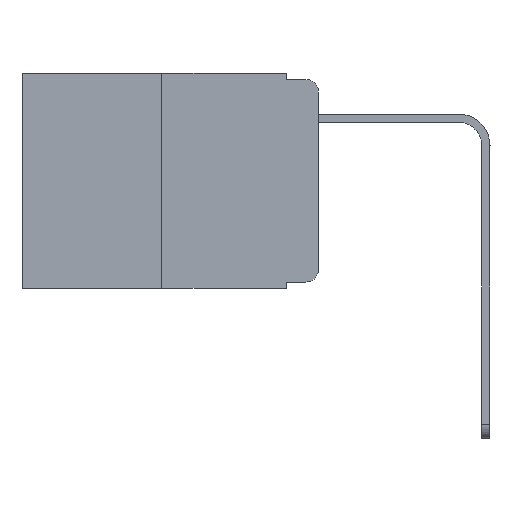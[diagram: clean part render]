
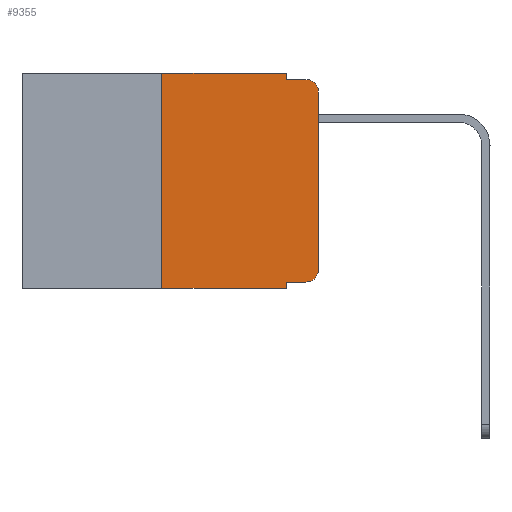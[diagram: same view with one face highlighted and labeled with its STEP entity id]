
A CAD part, left-side view. The second image highlights one B-rep face of the part: STEP entity #9355.
In plain terms, the highlighted planar face has unit normal (-1, 0, 0).
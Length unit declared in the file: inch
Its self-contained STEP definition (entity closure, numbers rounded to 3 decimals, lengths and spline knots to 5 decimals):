
#103 = VECTOR ( 'NONE', #19092, 39.37008 ) ;
#157 = EDGE_CURVE ( 'NONE', #6366, #18895, #11371, .T. ) ;
#1307 = VERTEX_POINT ( 'NONE', #1701 ) ;
#1343 = CARTESIAN_POINT ( 'NONE',  ( 0., 0.473, 0. ) ) ;
#1406 = DIRECTION ( 'NONE',  ( 0., -1., 0. ) ) ;
#1701 = CARTESIAN_POINT ( 'NONE',  ( 0., 0.25, 0. ) ) ;
#1942 = DIRECTION ( 'NONE',  ( -1., 0., 0. ) ) ;
#1989 = DIRECTION ( 'NONE',  ( -1., 0., 0. ) ) ;
#2503 = ORIENTED_EDGE ( 'NONE', *, *, #11614, .F. ) ;
#2694 = ORIENTED_EDGE ( 'NONE', *, *, #22215, .T. ) ;
#2781 = ORIENTED_EDGE ( 'NONE', *, *, #11770, .T. ) ;
#2900 = ORIENTED_EDGE ( 'NONE', *, *, #15340, .T. ) ;
#3020 = AXIS2_PLACEMENT_3D ( 'NONE', #21600, #1989, #19789 ) ;
#3275 = CARTESIAN_POINT ( 'NONE',  ( 0., 0.02, -0.333 ) ) ;
#3338 = DIRECTION ( 'NONE',  ( 0., 0., -1. ) ) ;
#3390 = LINE ( 'NONE', #14131, #22844 ) ;
#3753 = DIRECTION ( 'NONE',  ( 1., 0., 0. ) ) ;
#3938 = ORIENTED_EDGE ( 'NONE', *, *, #6670, .F. ) ;
#4120 = VECTOR ( 'NONE', #8656, 39.37008 ) ;
#4743 = AXIS2_PLACEMENT_3D ( 'NONE', #11235, #3753, #11484 ) ;
#4782 = VECTOR ( 'NONE', #10797, 39.37008 ) ;
#5432 = VECTOR ( 'NONE', #19909, 39.37008 ) ;
#5450 = ORIENTED_EDGE ( 'NONE', *, *, #157, .T. ) ;
#5679 = VERTEX_POINT ( 'NONE', #12437 ) ;
#6134 = VERTEX_POINT ( 'NONE', #3275 ) ;
#6366 = VERTEX_POINT ( 'NONE', #16719 ) ;
#6670 = EDGE_CURVE ( 'NONE', #13632, #20905, #15240, .T. ) ;
#7025 = ORIENTED_EDGE ( 'NONE', *, *, #9251, .F. ) ;
#7073 = ORIENTED_EDGE ( 'NONE', *, *, #15462, .F. ) ;
#7730 = CARTESIAN_POINT ( 'NONE',  ( 0., 0.25, -0.343 ) ) ;
#8656 = DIRECTION ( 'NONE',  ( 0., 0., -1. ) ) ;
#8911 = LINE ( 'NONE', #25001, #10462 ) ;
#9138 = EDGE_CURVE ( 'NONE', #13632, #6134, #19129, .T. ) ;
#9189 = ORIENTED_EDGE ( 'NONE', *, *, #9138, .T. ) ;
#9251 = EDGE_CURVE ( 'NONE', #23911, #1307, #3390, .T. ) ;
#9355 = ADVANCED_FACE ( 'NONE', ( #24097 ), #10888, .F. ) ;
#9690 = CARTESIAN_POINT ( 'NONE',  ( 0., 0.02, -0.03 ) ) ;
#10042 = CARTESIAN_POINT ( 'NONE',  ( 0., 0., 0. ) ) ;
#10237 = DIRECTION ( 'NONE',  ( 0., -1., 0. ) ) ;
#10462 = VECTOR ( 'NONE', #3338, 39.37008 ) ;
#10703 = CIRCLE ( 'NONE', #20778, 0.02 ) ;
#10740 = EDGE_CURVE ( 'NONE', #5679, #23069, #8911, .T. ) ;
#10797 = DIRECTION ( 'NONE',  ( 0., -1., 0. ) ) ;
#10888 = PLANE ( 'NONE',  #4743 ) ;
#11195 = CARTESIAN_POINT ( 'NONE',  ( 0., 0.051, 0. ) ) ;
#11235 = CARTESIAN_POINT ( 'NONE',  ( 0., 0.473, 0. ) ) ;
#11371 = LINE ( 'NONE', #10042, #5432 ) ;
#11484 = DIRECTION ( 'NONE',  ( 0., 0., -1. ) ) ;
#11614 = EDGE_CURVE ( 'NONE', #1307, #5679, #19893, .T. ) ;
#11694 = DIRECTION ( 'NONE',  ( 0., 0., -1. ) ) ;
#11770 = EDGE_CURVE ( 'NONE', #18895, #24451, #10703, .T. ) ;
#12437 = CARTESIAN_POINT ( 'NONE',  ( 0., 0.051, 0. ) ) ;
#12655 = VECTOR ( 'NONE', #1406, 39.37008 ) ;
#12814 = CARTESIAN_POINT ( 'NONE',  ( 0., 0.051, -0.333 ) ) ;
#13632 = VERTEX_POINT ( 'NONE', #12814 ) ;
#14131 = CARTESIAN_POINT ( 'NONE',  ( 0., 0.25, 0. ) ) ;
#15240 = LINE ( 'NONE', #11195, #4120 ) ;
#15340 = EDGE_CURVE ( 'NONE', #6134, #6366, #23103, .T. ) ;
#15462 = EDGE_CURVE ( 'NONE', #23069, #24451, #20326, .T. ) ;
#16719 = CARTESIAN_POINT ( 'NONE',  ( 0., 0., -0.313 ) ) ;
#17278 = DIRECTION ( 'NONE',  ( 0., 0., 1. ) ) ;
#17351 = CARTESIAN_POINT ( 'NONE',  ( 0., 0.051, -0.01 ) ) ;
#18026 = CARTESIAN_POINT ( 'NONE',  ( 0., 0.051, -0.343 ) ) ;
#18305 = ORIENTED_EDGE ( 'NONE', *, *, #10740, .F. ) ;
#18895 = VERTEX_POINT ( 'NONE', #23043 ) ;
#19092 = DIRECTION ( 'NONE',  ( 0., -1., 0. ) ) ;
#19129 = LINE ( 'NONE', #20832, #103 ) ;
#19789 = DIRECTION ( 'NONE',  ( 0., 0., -1. ) ) ;
#19893 = LINE ( 'NONE', #1343, #4782 ) ;
#19909 = DIRECTION ( 'NONE',  ( 0., 0., 1. ) ) ;
#20326 = LINE ( 'NONE', #17351, #12655 ) ;
#20778 = AXIS2_PLACEMENT_3D ( 'NONE', #9690, #1942, #11694 ) ;
#20832 = CARTESIAN_POINT ( 'NONE',  ( 0., 0.051, -0.333 ) ) ;
#20905 = VERTEX_POINT ( 'NONE', #18026 ) ;
#21256 = CARTESIAN_POINT ( 'NONE',  ( 0., 0.051, -0.01 ) ) ;
#21476 = EDGE_LOOP ( 'NONE', ( #5450, #2781, #7073, #18305, #2503, #7025, #2694, #3938, #9189, #2900 ) ) ;
#21600 = CARTESIAN_POINT ( 'NONE',  ( 0., 0.02, -0.313 ) ) ;
#22083 = CARTESIAN_POINT ( 'NONE',  ( 0., 0.473, -0.343 ) ) ;
#22215 = EDGE_CURVE ( 'NONE', #23911, #20905, #24282, .T. ) ;
#22844 = VECTOR ( 'NONE', #17278, 39.37008 ) ;
#23043 = CARTESIAN_POINT ( 'NONE',  ( 0., 0., -0.03 ) ) ;
#23069 = VERTEX_POINT ( 'NONE', #21256 ) ;
#23103 = CIRCLE ( 'NONE', #3020, 0.02 ) ;
#23911 = VERTEX_POINT ( 'NONE', #7730 ) ;
#24097 = FACE_OUTER_BOUND ( 'NONE', #21476, .T. ) ;
#24282 = LINE ( 'NONE', #22083, #25190 ) ;
#24451 = VERTEX_POINT ( 'NONE', #24698 ) ;
#24698 = CARTESIAN_POINT ( 'NONE',  ( 0., 0.02, -0.01 ) ) ;
#25001 = CARTESIAN_POINT ( 'NONE',  ( 0., 0.051, 0. ) ) ;
#25190 = VECTOR ( 'NONE', #10237, 39.37008 ) ;
